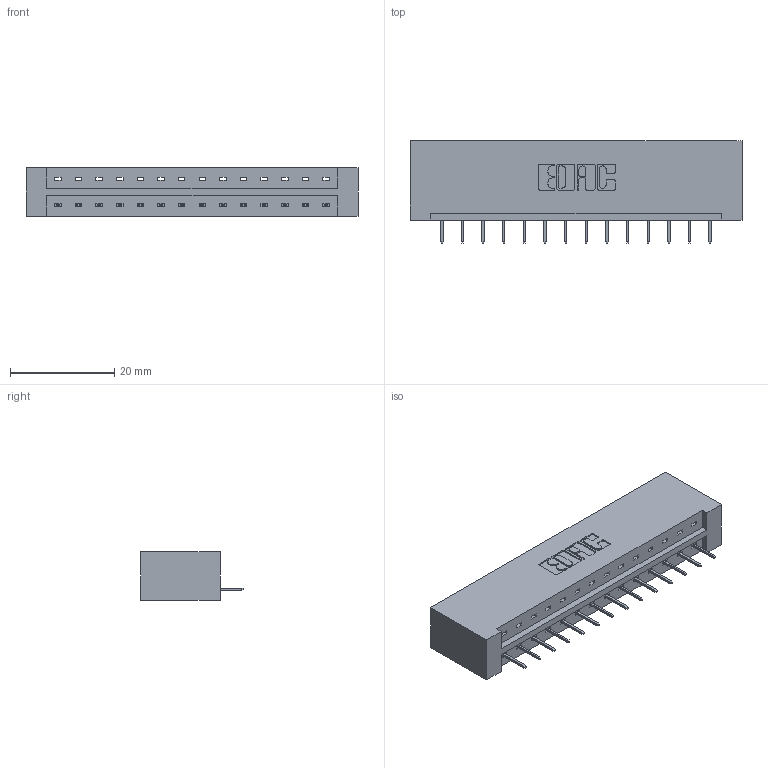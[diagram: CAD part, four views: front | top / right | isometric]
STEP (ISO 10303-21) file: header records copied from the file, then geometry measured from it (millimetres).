
FILE_DESCRIPTION (( 'STEP AP203' ), '1' );
FILE_NAME ('833-014-524-101.STEP', '2020-05-31T13:29:56', ( '' ), ( '' ), 'SwSTEP 2.0', 'SolidWorks 2020', '' );
FILE_SCHEMA (( 'CONFIG_CONTROL_DESIGN' ));
Length unit declared in the file: inch
Products named in the file (3): 345-292-001_345-293-124; 833-014-524-101; 833 Part_Lugless
Assembly tree (15 placements, depth 2):
  833-014-524-101
    833 Part_Lugless
    345-292-001_345-293-124  x14
Bounding box: 63.73 x 19.69 x 9.4 mm (x, y, z)
Volume: 6729.5 mm3; surface area: 6864.4 mm2
Topology: 15 solids, 15 shells, 974 faces, 2807 edges, 1814 vertices
Faces by surface type: plane 738, cylinder 236
Entity records: 11977 total; most frequent: CARTESIAN_POINT 2076, ORIENTED_EDGE 2026, DIRECTION 1801, EDGE_CURVE 1013, LINE 897, VECTOR 897, VERTEX_POINT 670, AXIS2_PLACEMENT_3D 452
